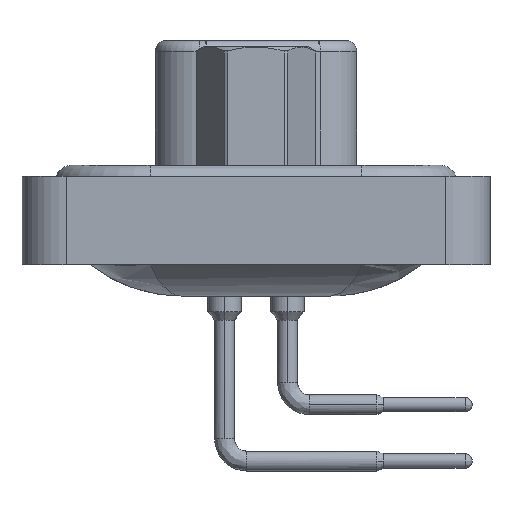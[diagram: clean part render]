
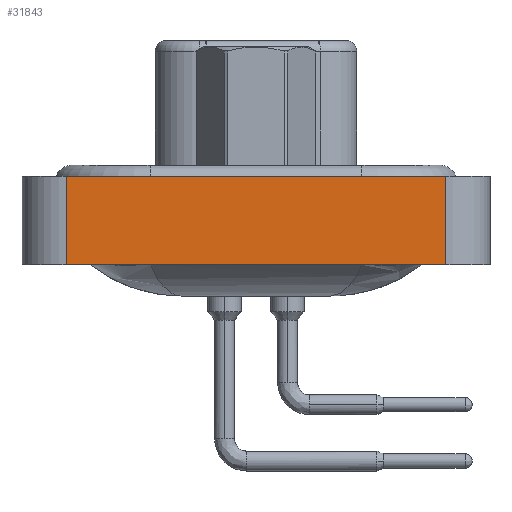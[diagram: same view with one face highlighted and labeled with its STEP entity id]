
A CAD part, left-side view. The second image highlights one B-rep face of the part: STEP entity #31843.
In plain terms, the highlighted planar face has unit normal (-1, 0, 0).
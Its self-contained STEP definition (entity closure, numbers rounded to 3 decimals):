
#2836 = EDGE_CURVE ( 'NONE', #26138, #12145, #20463, .T. ) ;
#3813 = CARTESIAN_POINT ( 'NONE',  ( -7.35, -8.55, 0.4 ) ) ;
#5163 = CARTESIAN_POINT ( 'NONE',  ( -7.35, -8.55, -3.6 ) ) ;
#5676 = ORIENTED_EDGE ( 'NONE', *, *, #32155, .F. ) ;
#5926 = DIRECTION ( 'NONE',  ( 0., 0., 1. ) ) ;
#6130 = LINE ( 'NONE', #3813, #12109 ) ;
#6377 = DIRECTION ( 'NONE',  ( 0., -1., 0. ) ) ;
#7248 = CARTESIAN_POINT ( 'NONE',  ( -7.35, 8.55, 0.4 ) ) ;
#10403 = DIRECTION ( 'NONE',  ( -1., 0., 0. ) ) ;
#10447 = CARTESIAN_POINT ( 'NONE',  ( -7.35, 8.55, -3.6 ) ) ;
#11056 = CARTESIAN_POINT ( 'NONE',  ( -7.35, -8.55, -3.6 ) ) ;
#11314 = EDGE_CURVE ( 'NONE', #12145, #15354, #25509, .T. ) ;
#12109 = VECTOR ( 'NONE', #29290, 1000. ) ;
#12145 = VERTEX_POINT ( 'NONE', #11056 ) ;
#13814 = FACE_OUTER_BOUND ( 'NONE', #16533, .T. ) ;
#14782 = ORIENTED_EDGE ( 'NONE', *, *, #2836, .T. ) ;
#15354 = VERTEX_POINT ( 'NONE', #29305 ) ;
#15886 = ORIENTED_EDGE ( 'NONE', *, *, #21928, .F. ) ;
#16533 = EDGE_LOOP ( 'NONE', ( #32120, #5676, #15886, #14782 ) ) ;
#20463 = LINE ( 'NONE', #29934, #25669 ) ;
#20577 = PLANE ( 'NONE',  #24669 ) ;
#21068 = VECTOR ( 'NONE', #5926, 1000. ) ;
#21870 = LINE ( 'NONE', #23835, #21068 ) ;
#21928 = EDGE_CURVE ( 'NONE', #26138, #29513, #21870, .T. ) ;
#23835 = CARTESIAN_POINT ( 'NONE',  ( -7.35, 8.55, -3.6 ) ) ;
#24669 = AXIS2_PLACEMENT_3D ( 'NONE', #5163, #10403, #28286 ) ;
#24705 = VECTOR ( 'NONE', #27109, 1000. ) ;
#25509 = LINE ( 'NONE', #27003, #24705 ) ;
#25669 = VECTOR ( 'NONE', #6377, 1000. ) ;
#26138 = VERTEX_POINT ( 'NONE', #10447 ) ;
#27003 = CARTESIAN_POINT ( 'NONE',  ( -7.35, -8.55, -3.6 ) ) ;
#27109 = DIRECTION ( 'NONE',  ( 0., 0., 1. ) ) ;
#28286 = DIRECTION ( 'NONE',  ( 0., 0., 1. ) ) ;
#29290 = DIRECTION ( 'NONE',  ( 0., -1., 0. ) ) ;
#29305 = CARTESIAN_POINT ( 'NONE',  ( -7.35, -8.55, 0.4 ) ) ;
#29513 = VERTEX_POINT ( 'NONE', #7248 ) ;
#29934 = CARTESIAN_POINT ( 'NONE',  ( -7.35, -8.55, -3.6 ) ) ;
#31843 = ADVANCED_FACE ( 'NONE', ( #13814 ), #20577, .T. ) ;
#32120 = ORIENTED_EDGE ( 'NONE', *, *, #11314, .T. ) ;
#32155 = EDGE_CURVE ( 'NONE', #29513, #15354, #6130, .T. ) ;
